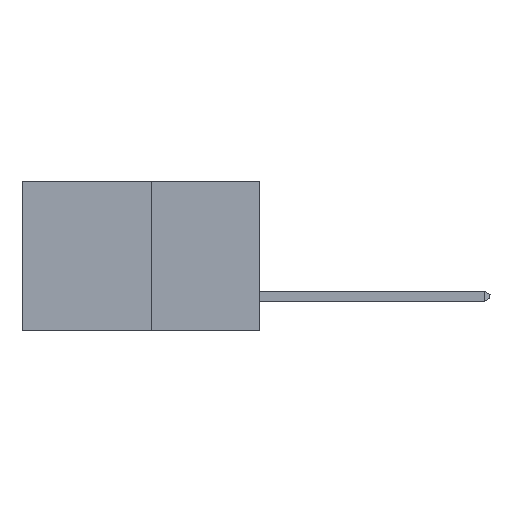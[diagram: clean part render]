
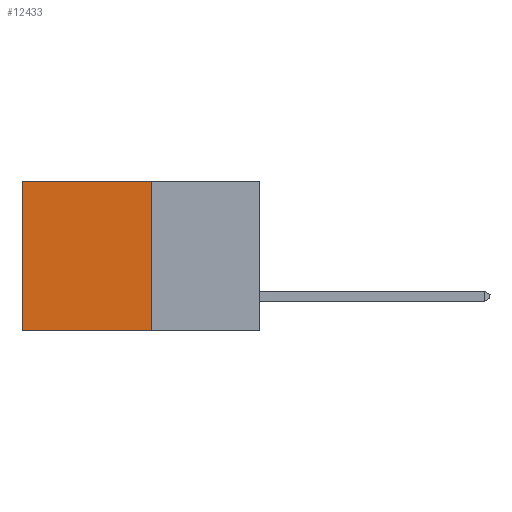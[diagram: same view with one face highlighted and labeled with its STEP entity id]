
A CAD part, left-side view. The second image highlights one B-rep face of the part: STEP entity #12433.
In plain terms, the highlighted planar face has unit normal (-1, 0, 0).
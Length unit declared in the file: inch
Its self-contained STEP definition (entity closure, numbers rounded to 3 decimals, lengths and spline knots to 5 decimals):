
#276 = VERTEX_POINT ( 'NONE', #10810 ) ;
#867 = ORIENTED_EDGE ( 'NONE', *, *, #4421, .F. ) ;
#998 = CARTESIAN_POINT ( 'NONE',  ( 0.277, 0.27, -0.37 ) ) ;
#1213 = ORIENTED_EDGE ( 'NONE', *, *, #3224, .F. ) ;
#1267 = CARTESIAN_POINT ( 'NONE',  ( 0.277, 0.27, -0.37 ) ) ;
#1324 = LINE ( 'NONE', #998, #4139 ) ;
#1951 = ORIENTED_EDGE ( 'NONE', *, *, #3107, .T. ) ;
#2089 = CARTESIAN_POINT ( 'NONE',  ( 0.277, 0.59, -0.37 ) ) ;
#2840 = VERTEX_POINT ( 'NONE', #2089 ) ;
#3107 = EDGE_CURVE ( 'NONE', #276, #9366, #11323, .T. ) ;
#3224 = EDGE_CURVE ( 'NONE', #10363, #2840, #1324, .T. ) ;
#3893 = ORIENTED_EDGE ( 'NONE', *, *, #7538, .T. ) ;
#3929 = LINE ( 'NONE', #9699, #6336 ) ;
#4004 = LINE ( 'NONE', #4182, #8797 ) ;
#4139 = VECTOR ( 'NONE', #9763, 39.37008 ) ;
#4161 = DIRECTION ( 'NONE',  ( 0., 0., -1. ) ) ;
#4182 = CARTESIAN_POINT ( 'NONE',  ( 0.277, 0.59, -0.37 ) ) ;
#4421 = EDGE_CURVE ( 'NONE', #276, #10363, #3929, .T. ) ;
#4461 = PLANE ( 'NONE',  #4668 ) ;
#4668 = AXIS2_PLACEMENT_3D ( 'NONE', #1267, #5490, #12259 ) ;
#5490 = DIRECTION ( 'NONE',  ( 1., 0., 0. ) ) ;
#5999 = FACE_OUTER_BOUND ( 'NONE', #9975, .T. ) ;
#6336 = VECTOR ( 'NONE', #6571, 39.37008 ) ;
#6571 = DIRECTION ( 'NONE',  ( 0., 0., -1. ) ) ;
#7538 = EDGE_CURVE ( 'NONE', #9366, #2840, #4004, .T. ) ;
#8489 = VECTOR ( 'NONE', #11504, 39.37008 ) ;
#8797 = VECTOR ( 'NONE', #4161, 39.37008 ) ;
#9366 = VERTEX_POINT ( 'NONE', #11053 ) ;
#9699 = CARTESIAN_POINT ( 'NONE',  ( 0.277, 0.27, -0.37 ) ) ;
#9763 = DIRECTION ( 'NONE',  ( 0., 1., 0. ) ) ;
#9975 = EDGE_LOOP ( 'NONE', ( #3893, #1213, #867, #1951 ) ) ;
#10363 = VERTEX_POINT ( 'NONE', #12504 ) ;
#10810 = CARTESIAN_POINT ( 'NONE',  ( 0.277, 0.27, 0. ) ) ;
#11053 = CARTESIAN_POINT ( 'NONE',  ( 0.277, 0.59, 0. ) ) ;
#11323 = LINE ( 'NONE', #11391, #8489 ) ;
#11391 = CARTESIAN_POINT ( 'NONE',  ( 0.277, 0.27, 0. ) ) ;
#11504 = DIRECTION ( 'NONE',  ( 0., 1., 0. ) ) ;
#12259 = DIRECTION ( 'NONE',  ( 0., 0., -1. ) ) ;
#12433 = ADVANCED_FACE ( 'NONE', ( #5999 ), #4461, .F. ) ;
#12504 = CARTESIAN_POINT ( 'NONE',  ( 0.277, 0.27, -0.37 ) ) ;
